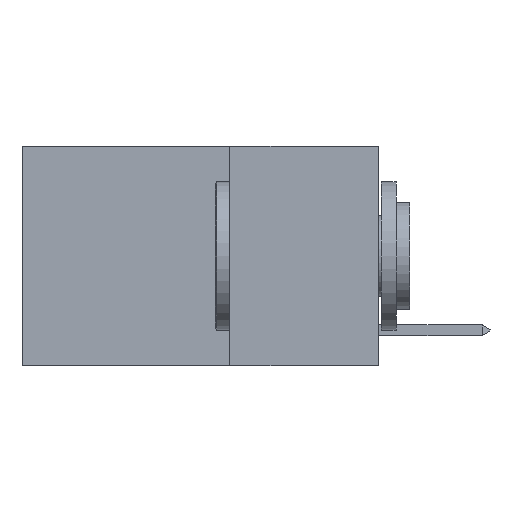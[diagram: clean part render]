
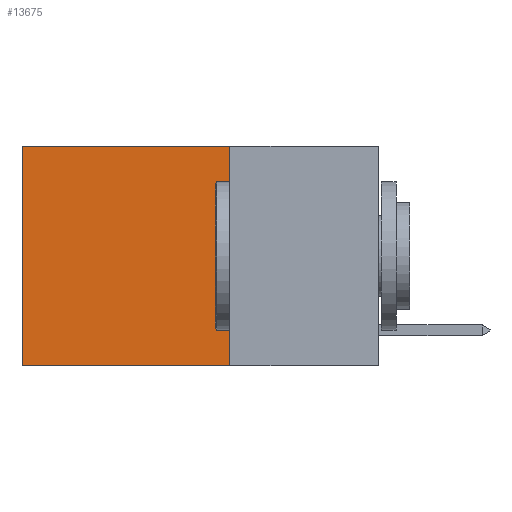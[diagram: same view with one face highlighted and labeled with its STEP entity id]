
A CAD part, left-side view. The second image highlights one B-rep face of the part: STEP entity #13675.
In plain terms, the highlighted planar face has unit normal (-1, 0, 0).
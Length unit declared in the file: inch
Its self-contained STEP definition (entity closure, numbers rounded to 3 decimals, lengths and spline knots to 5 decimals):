
#468 = CARTESIAN_POINT ( 'NONE',  ( 0.2625, 0.25, 0. ) ) ;
#1343 = CARTESIAN_POINT ( 'NONE',  ( 0.2625, 0.25, 0. ) ) ;
#2008 = EDGE_CURVE ( 'NONE', #14965, #19064, #13369, .T. ) ;
#2189 = DIRECTION ( 'NONE',  ( 0., 0., -1. ) ) ;
#2299 = EDGE_CURVE ( 'NONE', #6772, #19064, #10610, .T. ) ;
#3006 = FACE_OUTER_BOUND ( 'NONE', #16391, .T. ) ;
#3850 = ORIENTED_EDGE ( 'NONE', *, *, #5153, .F. ) ;
#3868 = ORIENTED_EDGE ( 'NONE', *, *, #2008, .F. ) ;
#4632 = ORIENTED_EDGE ( 'NONE', *, *, #21737, .T. ) ;
#4941 = DIRECTION ( 'NONE',  ( 0., 1., 0. ) ) ;
#5153 = EDGE_CURVE ( 'NONE', #10372, #14965, #21178, .T. ) ;
#5642 = DIRECTION ( 'NONE',  ( 0., 1., 0. ) ) ;
#5660 = VECTOR ( 'NONE', #5642, 39.37008 ) ;
#6289 = CARTESIAN_POINT ( 'NONE',  ( 0.2625, 0.25, 0. ) ) ;
#6772 = VERTEX_POINT ( 'NONE', #21687 ) ;
#6846 = VECTOR ( 'NONE', #9302, 39.37008 ) ;
#7271 = CARTESIAN_POINT ( 'NONE',  ( 0.2625, 0.6, 0. ) ) ;
#8060 = DIRECTION ( 'NONE',  ( 0., 0., -1. ) ) ;
#9302 = DIRECTION ( 'NONE',  ( 0., 0., -1. ) ) ;
#9801 = VECTOR ( 'NONE', #2189, 39.37008 ) ;
#10372 = VERTEX_POINT ( 'NONE', #13090 ) ;
#10607 = CARTESIAN_POINT ( 'NONE',  ( 0.2625, 0.25, -0.37 ) ) ;
#10610 = LINE ( 'NONE', #7271, #9801 ) ;
#13090 = CARTESIAN_POINT ( 'NONE',  ( 0.2625, 0.25, 0. ) ) ;
#13369 = LINE ( 'NONE', #20163, #21238 ) ;
#13675 = ADVANCED_FACE ( 'NONE', ( #3006 ), #19985, .F. ) ;
#13767 = LINE ( 'NONE', #468, #5660 ) ;
#14965 = VERTEX_POINT ( 'NONE', #10607 ) ;
#16391 = EDGE_LOOP ( 'NONE', ( #18381, #3868, #3850, #4632 ) ) ;
#18381 = ORIENTED_EDGE ( 'NONE', *, *, #2299, .T. ) ;
#19064 = VERTEX_POINT ( 'NONE', #21209 ) ;
#19762 = DIRECTION ( 'NONE',  ( 1., 0., 0. ) ) ;
#19985 = PLANE ( 'NONE',  #21143 ) ;
#20163 = CARTESIAN_POINT ( 'NONE',  ( 0.2625, 0.25, -0.37 ) ) ;
#21143 = AXIS2_PLACEMENT_3D ( 'NONE', #1343, #19762, #8060 ) ;
#21178 = LINE ( 'NONE', #6289, #6846 ) ;
#21209 = CARTESIAN_POINT ( 'NONE',  ( 0.2625, 0.6, -0.37 ) ) ;
#21238 = VECTOR ( 'NONE', #4941, 39.37008 ) ;
#21687 = CARTESIAN_POINT ( 'NONE',  ( 0.2625, 0.6, 0. ) ) ;
#21737 = EDGE_CURVE ( 'NONE', #10372, #6772, #13767, .T. ) ;
